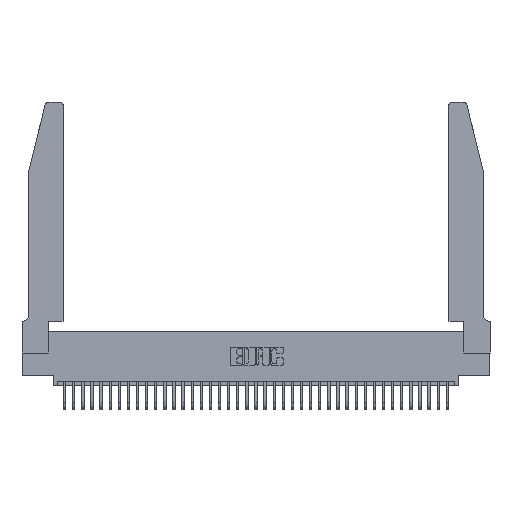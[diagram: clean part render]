
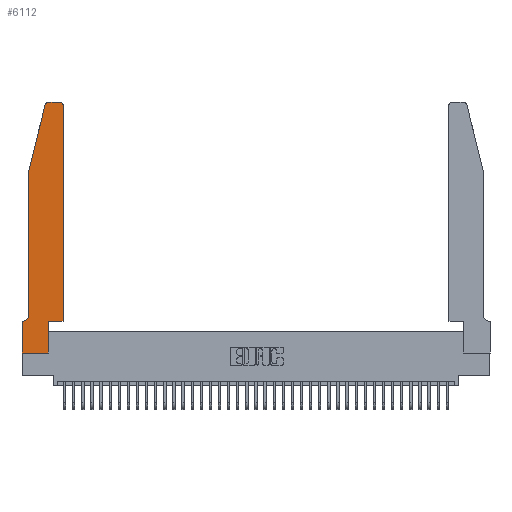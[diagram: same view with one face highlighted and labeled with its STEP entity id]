
A CAD part, top view. The second image highlights one B-rep face of the part: STEP entity #6112.
In plain terms, the highlighted planar face has unit normal (0, 0, 1).
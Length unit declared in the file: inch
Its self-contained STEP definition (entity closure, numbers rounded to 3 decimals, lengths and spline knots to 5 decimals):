
#82 = ORIENTED_EDGE ( 'NONE', *, *, #3758, .T. ) ;
#86 = AXIS2_PLACEMENT_3D ( 'NONE', #19194, #3659, #25396 ) ;
#390 = EDGE_CURVE ( 'NONE', #8208, #40074, #1196, .T. ) ;
#820 = DIRECTION ( 'NONE',  ( 1., 0., 0. ) ) ;
#891 = CIRCLE ( 'NONE', #19229, 0.03 ) ;
#1196 = LINE ( 'NONE', #30180, #32294 ) ;
#1406 = VECTOR ( 'NONE', #17988, 39.37008 ) ;
#1612 = DIRECTION ( 'NONE',  ( -0.239, -0.971, 0. ) ) ;
#1987 = DIRECTION ( 'NONE',  ( 0., 1., 0. ) ) ;
#2418 = LINE ( 'NONE', #33368, #1406 ) ;
#3167 = CARTESIAN_POINT ( 'NONE',  ( 0.0755, 0.35, 0.37 ) ) ;
#3520 = CARTESIAN_POINT ( 'NONE',  ( 0.284, 2.75, 0.37 ) ) ;
#3659 = DIRECTION ( 'NONE',  ( 0., 0., 1. ) ) ;
#3758 = EDGE_CURVE ( 'NONE', #13943, #34115, #2418, .T. ) ;
#3963 = VERTEX_POINT ( 'NONE', #6556 ) ;
#4007 = LINE ( 'NONE', #26529, #19593 ) ;
#4111 = VERTEX_POINT ( 'NONE', #13514 ) ;
#4352 = LINE ( 'NONE', #4470, #20906 ) ;
#4470 = CARTESIAN_POINT ( 'NONE',  ( 0., 0., 0.37 ) ) ;
#4543 = ORIENTED_EDGE ( 'NONE', *, *, #390, .T. ) ;
#5466 = VECTOR ( 'NONE', #36070, 39.37008 ) ;
#5709 = CARTESIAN_POINT ( 'NONE',  ( 0.284, 2.72, 0.37 ) ) ;
#5939 = CARTESIAN_POINT ( 'NONE',  ( 0.0755, 0.42, 0.37 ) ) ;
#6112 = ADVANCED_FACE ( 'NONE', ( #23990 ), #9798, .T. ) ;
#6556 = CARTESIAN_POINT ( 'NONE',  ( 0.4505, 2.72, 0.37 ) ) ;
#7603 = VERTEX_POINT ( 'NONE', #16638 ) ;
#7626 = LINE ( 'NONE', #12560, #15910 ) ;
#7808 = EDGE_CURVE ( 'NONE', #31282, #8208, #38353, .T. ) ;
#8022 = ORIENTED_EDGE ( 'NONE', *, *, #7808, .T. ) ;
#8208 = VERTEX_POINT ( 'NONE', #19309 ) ;
#8841 = DIRECTION ( 'NONE',  ( 1., 0., 0. ) ) ;
#9060 = EDGE_CURVE ( 'NONE', #16238, #3963, #24773, .T. ) ;
#9145 = DIRECTION ( 'NONE',  ( 0., 0., -1. ) ) ;
#9407 = DIRECTION ( 'NONE',  ( 1., 0., 0. ) ) ;
#9798 = PLANE ( 'NONE',  #86 ) ;
#10043 = ORIENTED_EDGE ( 'NONE', *, *, #37693, .T. ) ;
#10382 = VERTEX_POINT ( 'NONE', #14223 ) ;
#11045 = EDGE_CURVE ( 'NONE', #36273, #10382, #23653, .T. ) ;
#11601 = ORIENTED_EDGE ( 'NONE', *, *, #30750, .T. ) ;
#12340 = AXIS2_PLACEMENT_3D ( 'NONE', #5709, #27419, #8841 ) ;
#12560 = CARTESIAN_POINT ( 'NONE',  ( 0.4505, 0.35, 0.37 ) ) ;
#12762 = AXIS2_PLACEMENT_3D ( 'NONE', #27724, #9145, #30823 ) ;
#13451 = VECTOR ( 'NONE', #21939, 39.37008 ) ;
#13514 = CARTESIAN_POINT ( 'NONE',  ( 0., 0.35, 0.37 ) ) ;
#13902 = CARTESIAN_POINT ( 'NONE',  ( 0.0055, 0.35, 0.37 ) ) ;
#13943 = VERTEX_POINT ( 'NONE', #21259 ) ;
#14223 = CARTESIAN_POINT ( 'NONE',  ( 0.25487, 2.72718, 0.37 ) ) ;
#15910 = VECTOR ( 'NONE', #9407, 39.37008 ) ;
#16048 = LINE ( 'NONE', #40123, #39655 ) ;
#16075 = CARTESIAN_POINT ( 'NONE',  ( 0.4505, 0.35, 0.37 ) ) ;
#16238 = VERTEX_POINT ( 'NONE', #16075 ) ;
#16638 = CARTESIAN_POINT ( 'NONE',  ( 0.4205, 2.75, 0.37 ) ) ;
#16805 = EDGE_CURVE ( 'NONE', #7603, #36273, #16048, .T. ) ;
#17557 = CARTESIAN_POINT ( 'NONE',  ( 0., 0., 0.37 ) ) ;
#17873 = DIRECTION ( 'NONE',  ( 0., 1., 0. ) ) ;
#17988 = DIRECTION ( 'NONE',  ( 0., -1., 0. ) ) ;
#18291 = ORIENTED_EDGE ( 'NONE', *, *, #21289, .T. ) ;
#19194 = CARTESIAN_POINT ( 'NONE',  ( 0., 0.35, 0.37 ) ) ;
#19229 = AXIS2_PLACEMENT_3D ( 'NONE', #37994, #19554, #820 ) ;
#19309 = CARTESIAN_POINT ( 'NONE',  ( 0.2865, 0., 0.37 ) ) ;
#19554 = DIRECTION ( 'NONE',  ( 0., 0., 1. ) ) ;
#19593 = VECTOR ( 'NONE', #1612, 39.37008 ) ;
#20744 = ORIENTED_EDGE ( 'NONE', *, *, #31779, .T. ) ;
#20906 = VECTOR ( 'NONE', #29295, 39.37008 ) ;
#21259 = CARTESIAN_POINT ( 'NONE',  ( 0.0755, 2., 0.37 ) ) ;
#21289 = EDGE_CURVE ( 'NONE', #4111, #31282, #4352, .T. ) ;
#21939 = DIRECTION ( 'NONE',  ( -1., 0., 0. ) ) ;
#23653 = CIRCLE ( 'NONE', #12340, 0.03 ) ;
#23990 = FACE_OUTER_BOUND ( 'NONE', #35132, .T. ) ;
#24773 = LINE ( 'NONE', #36048, #40155 ) ;
#24811 = DIRECTION ( 'NONE',  ( -1., 0., 0. ) ) ;
#24921 = CARTESIAN_POINT ( 'NONE',  ( 0., 0., 0.37 ) ) ;
#25396 = DIRECTION ( 'NONE',  ( 1., 0., 0. ) ) ;
#25488 = ORIENTED_EDGE ( 'NONE', *, *, #11045, .T. ) ;
#25891 = ORIENTED_EDGE ( 'NONE', *, *, #9060, .T. ) ;
#26002 = ORIENTED_EDGE ( 'NONE', *, *, #28031, .T. ) ;
#26529 = CARTESIAN_POINT ( 'NONE',  ( 0.0755, 2., 0.37 ) ) ;
#27419 = DIRECTION ( 'NONE',  ( 0., 0., 1. ) ) ;
#27724 = CARTESIAN_POINT ( 'NONE',  ( 0.0055, 0.42, 0.37 ) ) ;
#28031 = EDGE_CURVE ( 'NONE', #40074, #16238, #7626, .T. ) ;
#29295 = DIRECTION ( 'NONE',  ( 0., -1., 0. ) ) ;
#30180 = CARTESIAN_POINT ( 'NONE',  ( 0.2865, 0.35, 0.37 ) ) ;
#30750 = EDGE_CURVE ( 'NONE', #3963, #7603, #891, .T. ) ;
#30823 = DIRECTION ( 'NONE',  ( -1., 0., 0. ) ) ;
#31282 = VERTEX_POINT ( 'NONE', #24921 ) ;
#31779 = EDGE_CURVE ( 'NONE', #34115, #36497, #34341, .T. ) ;
#32294 = VECTOR ( 'NONE', #17873, 39.37008 ) ;
#33368 = CARTESIAN_POINT ( 'NONE',  ( 0.0755, 2., 0.37 ) ) ;
#34115 = VERTEX_POINT ( 'NONE', #5939 ) ;
#34202 = EDGE_CURVE ( 'NONE', #36497, #4111, #38036, .T. ) ;
#34341 = CIRCLE ( 'NONE', #12762, 0.07 ) ;
#35132 = EDGE_LOOP ( 'NONE', ( #37087, #25488, #10043, #82, #20744, #36699, #18291, #8022, #4543, #26002, #25891, #11601 ) ) ;
#36048 = CARTESIAN_POINT ( 'NONE',  ( 0.4505, 0.35, 0.37 ) ) ;
#36070 = DIRECTION ( 'NONE',  ( 1., 0., 0. ) ) ;
#36273 = VERTEX_POINT ( 'NONE', #3520 ) ;
#36497 = VERTEX_POINT ( 'NONE', #13902 ) ;
#36699 = ORIENTED_EDGE ( 'NONE', *, *, #34202, .T. ) ;
#37087 = ORIENTED_EDGE ( 'NONE', *, *, #16805, .T. ) ;
#37693 = EDGE_CURVE ( 'NONE', #10382, #13943, #4007, .T. ) ;
#37701 = CARTESIAN_POINT ( 'NONE',  ( 0.2865, 0.35, 0.37 ) ) ;
#37994 = CARTESIAN_POINT ( 'NONE',  ( 0.4205, 2.72, 0.37 ) ) ;
#38036 = LINE ( 'NONE', #3167, #13451 ) ;
#38353 = LINE ( 'NONE', #17557, #5466 ) ;
#39655 = VECTOR ( 'NONE', #24811, 39.37008 ) ;
#40074 = VERTEX_POINT ( 'NONE', #37701 ) ;
#40123 = CARTESIAN_POINT ( 'NONE',  ( 0.2605, 2.75, 0.37 ) ) ;
#40155 = VECTOR ( 'NONE', #1987, 39.37008 ) ;
